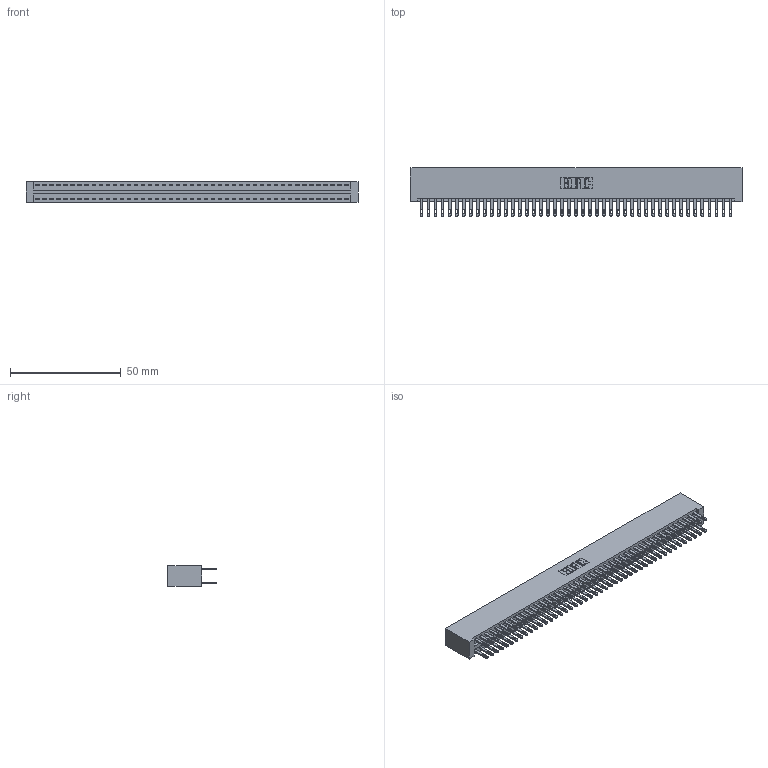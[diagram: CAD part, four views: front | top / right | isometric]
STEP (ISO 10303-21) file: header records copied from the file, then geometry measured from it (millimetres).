
FILE_DESCRIPTION (( 'STEP AP203' ), '1' );
FILE_NAME ('346-090-500-201.STEP', '2022-05-26T02:44:43', ( '' ), ( '' ), 'SwSTEP 2.0', 'SolidWorks 2020', '' );
FILE_SCHEMA (( 'CONFIG_CONTROL_DESIGN' ));
Length unit declared in the file: inch
Products named in the file (3): 345-292-001_345-293-100; 346 Part_No Mounting Lugs; 346-090-500-201
Assembly tree (91 placements, depth 2):
  346-090-500-201
    346 Part_No Mounting Lugs
    345-292-001_345-293-100  x90
Bounding box: 150.11 x 21.84 x 9.4 mm (x, y, z)
Volume: 15509.6 mm3; surface area: 22471.3 mm2
Topology: 91 solids, 91 shells, 4434 faces, 13535 edges, 9022 vertices
Faces by surface type: plane 2682, cylinder 1752
Entity records: 28617 total; most frequent: CARTESIAN_POINT 4708, ORIENTED_EDGE 4642, DIRECTION 4197, EDGE_CURVE 2321, VECTOR 2013, LINE 2013, VERTEX_POINT 1546, AXIS2_PLACEMENT_3D 1092
